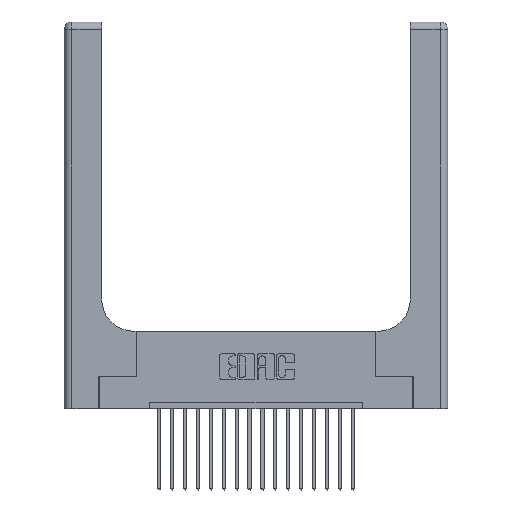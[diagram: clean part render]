
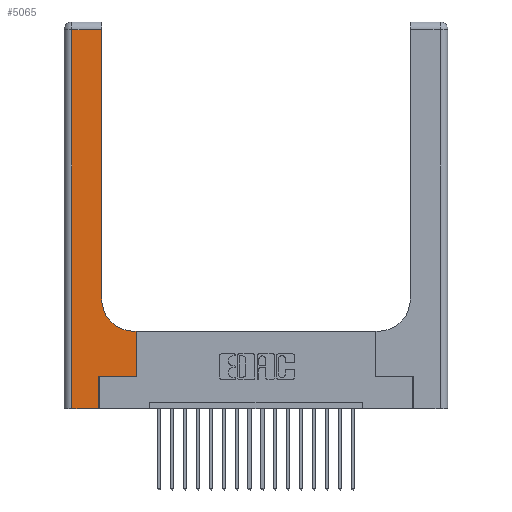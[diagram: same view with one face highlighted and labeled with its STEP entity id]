
A CAD part, top view. The second image highlights one B-rep face of the part: STEP entity #5065.
In plain terms, the highlighted planar face has unit normal (0, 0, 1).
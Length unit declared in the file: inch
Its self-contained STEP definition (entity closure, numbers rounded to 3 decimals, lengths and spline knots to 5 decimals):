
#387 = VERTEX_POINT ( 'NONE', #7708 ) ;
#529 = CARTESIAN_POINT ( 'NONE',  ( 0., 3., 0.37 ) ) ;
#708 = VERTEX_POINT ( 'NONE', #15833 ) ;
#879 = ORIENTED_EDGE ( 'NONE', *, *, #1054, .T. ) ;
#1054 = EDGE_CURVE ( 'NONE', #6096, #18811, #12624, .T. ) ;
#1133 = DIRECTION ( 'NONE',  ( 1., 0., 0. ) ) ;
#1514 = CARTESIAN_POINT ( 'NONE',  ( 0.2915, 2.94, 0.37 ) ) ;
#1677 = VECTOR ( 'NONE', #10142, 39.37008 ) ;
#2018 = ORIENTED_EDGE ( 'NONE', *, *, #7782, .T. ) ;
#2127 = AXIS2_PLACEMENT_3D ( 'NONE', #2546, #10761, #1133 ) ;
#2230 = LINE ( 'NONE', #9413, #10268 ) ;
#2546 = CARTESIAN_POINT ( 'NONE',  ( 0.5415, 0.85, 0.37 ) ) ;
#3029 = CARTESIAN_POINT ( 'NONE',  ( 0.5585, 0.25, 0.37 ) ) ;
#3357 = CARTESIAN_POINT ( 'NONE',  ( 0.2915, 3., 0.37 ) ) ;
#3555 = VECTOR ( 'NONE', #14007, 39.37008 ) ;
#3676 = CARTESIAN_POINT ( 'NONE',  ( 0.2915, 0.85, 0.37 ) ) ;
#3684 = EDGE_CURVE ( 'NONE', #5698, #12921, #10540, .T. ) ;
#3854 = VECTOR ( 'NONE', #4101, 39.37008 ) ;
#3905 = EDGE_LOOP ( 'NONE', ( #10927, #8390, #9927, #15704, #2018, #879, #17670, #20418, #15047 ) ) ;
#4101 = DIRECTION ( 'NONE',  ( 1., 0., 0. ) ) ;
#4648 = LINE ( 'NONE', #15353, #8667 ) ;
#5065 = ADVANCED_FACE ( 'NONE', ( #16271 ), #16566, .F. ) ;
#5153 = DIRECTION ( 'NONE',  ( 0., 0., -1. ) ) ;
#5249 = VECTOR ( 'NONE', #9814, 39.37008 ) ;
#5421 = EDGE_CURVE ( 'NONE', #12921, #708, #2230, .T. ) ;
#5688 = LINE ( 'NONE', #19503, #1677 ) ;
#5698 = VERTEX_POINT ( 'NONE', #10120 ) ;
#5764 = DIRECTION ( 'NONE',  ( 0., 1., 0. ) ) ;
#5814 = LINE ( 'NONE', #3357, #3555 ) ;
#6096 = VERTEX_POINT ( 'NONE', #17932 ) ;
#6402 = DIRECTION ( 'NONE',  ( 1., 0., 0. ) ) ;
#7149 = EDGE_CURVE ( 'NONE', #18811, #9536, #13173, .T. ) ;
#7708 = CARTESIAN_POINT ( 'NONE',  ( 0.5415, 0.6, 0.37 ) ) ;
#7782 = EDGE_CURVE ( 'NONE', #708, #6096, #4648, .T. ) ;
#8390 = ORIENTED_EDGE ( 'NONE', *, *, #13679, .T. ) ;
#8636 = LINE ( 'NONE', #16844, #10670 ) ;
#8667 = VECTOR ( 'NONE', #5764, 39.37008 ) ;
#8685 = VERTEX_POINT ( 'NONE', #1514 ) ;
#9413 = CARTESIAN_POINT ( 'NONE',  ( 0., 0., 0.37 ) ) ;
#9536 = VERTEX_POINT ( 'NONE', #13249 ) ;
#9814 = DIRECTION ( 'NONE',  ( 0., -1., 0. ) ) ;
#9911 = CARTESIAN_POINT ( 'NONE',  ( 0.5585, 0.25, 0.37 ) ) ;
#9927 = ORIENTED_EDGE ( 'NONE', *, *, #3684, .T. ) ;
#10120 = CARTESIAN_POINT ( 'NONE',  ( 0.06, 2.94, 0.37 ) ) ;
#10142 = DIRECTION ( 'NONE',  ( -1., 0., 0. ) ) ;
#10268 = VECTOR ( 'NONE', #6402, 39.37008 ) ;
#10540 = LINE ( 'NONE', #11414, #5249 ) ;
#10578 = DIRECTION ( 'NONE',  ( -1., 0., 0. ) ) ;
#10650 = CARTESIAN_POINT ( 'NONE',  ( 0.269, 0.25, 0.37 ) ) ;
#10670 = VECTOR ( 'NONE', #10578, 39.37008 ) ;
#10761 = DIRECTION ( 'NONE',  ( 0., 0., -1. ) ) ;
#10927 = ORIENTED_EDGE ( 'NONE', *, *, #16092, .T. ) ;
#11414 = CARTESIAN_POINT ( 'NONE',  ( 0.06, 3., 0.37 ) ) ;
#12388 = EDGE_CURVE ( 'NONE', #9536, #387, #5688, .T. ) ;
#12406 = VERTEX_POINT ( 'NONE', #3676 ) ;
#12488 = DIRECTION ( 'NONE',  ( 0., 1., 0. ) ) ;
#12624 = LINE ( 'NONE', #10650, #3854 ) ;
#12712 = EDGE_CURVE ( 'NONE', #387, #12406, #18705, .T. ) ;
#12921 = VERTEX_POINT ( 'NONE', #14727 ) ;
#13173 = LINE ( 'NONE', #3029, #17454 ) ;
#13249 = CARTESIAN_POINT ( 'NONE',  ( 0.5585, 0.6, 0.37 ) ) ;
#13679 = EDGE_CURVE ( 'NONE', #8685, #5698, #8636, .T. ) ;
#14007 = DIRECTION ( 'NONE',  ( 0., 1., 0. ) ) ;
#14727 = CARTESIAN_POINT ( 'NONE',  ( 0.06, 0., 0.37 ) ) ;
#15047 = ORIENTED_EDGE ( 'NONE', *, *, #12712, .T. ) ;
#15353 = CARTESIAN_POINT ( 'NONE',  ( 0.269, 0., 0.37 ) ) ;
#15704 = ORIENTED_EDGE ( 'NONE', *, *, #5421, .T. ) ;
#15833 = CARTESIAN_POINT ( 'NONE',  ( 0.269, 0., 0.37 ) ) ;
#16092 = EDGE_CURVE ( 'NONE', #12406, #8685, #5814, .T. ) ;
#16271 = FACE_OUTER_BOUND ( 'NONE', #3905, .T. ) ;
#16566 = PLANE ( 'NONE',  #19904 ) ;
#16844 = CARTESIAN_POINT ( 'NONE',  ( 0., 2.94, 0.37 ) ) ;
#17454 = VECTOR ( 'NONE', #12488, 39.37008 ) ;
#17670 = ORIENTED_EDGE ( 'NONE', *, *, #7149, .T. ) ;
#17932 = CARTESIAN_POINT ( 'NONE',  ( 0.269, 0.25, 0.37 ) ) ;
#18047 = DIRECTION ( 'NONE',  ( -1., 0., 0. ) ) ;
#18705 = CIRCLE ( 'NONE', #2127, 0.25 ) ;
#18811 = VERTEX_POINT ( 'NONE', #9911 ) ;
#19503 = CARTESIAN_POINT ( 'NONE',  ( 0.2915, 0.6, 0.37 ) ) ;
#19904 = AXIS2_PLACEMENT_3D ( 'NONE', #529, #5153, #18047 ) ;
#20418 = ORIENTED_EDGE ( 'NONE', *, *, #12388, .T. ) ;
